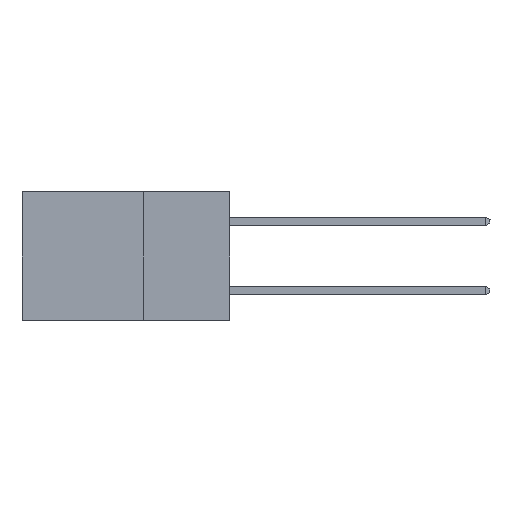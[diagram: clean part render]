
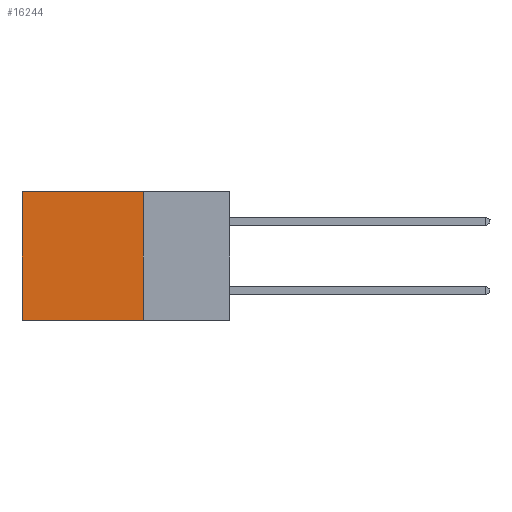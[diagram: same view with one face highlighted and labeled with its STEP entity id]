
A CAD part, left-side view. The second image highlights one B-rep face of the part: STEP entity #16244.
In plain terms, the highlighted planar face has unit normal (-1, 0, 0).
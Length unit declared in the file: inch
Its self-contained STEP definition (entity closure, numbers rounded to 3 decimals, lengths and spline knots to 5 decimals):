
#176 = FACE_OUTER_BOUND ( 'NONE', #15796, .T. ) ;
#634 = VECTOR ( 'NONE', #16103, 39.37008 ) ;
#1981 = ORIENTED_EDGE ( 'NONE', *, *, #16188, .T. ) ;
#2807 = CARTESIAN_POINT ( 'NONE',  ( 0.2615, 0.25, 0. ) ) ;
#4240 = DIRECTION ( 'NONE',  ( 1., 0., 0. ) ) ;
#4374 = LINE ( 'NONE', #25330, #18898 ) ;
#4398 = EDGE_CURVE ( 'NONE', #14959, #13245, #10798, .T. ) ;
#4508 = PLANE ( 'NONE',  #19746 ) ;
#4980 = DIRECTION ( 'NONE',  ( 0., 0., -1. ) ) ;
#7429 = VECTOR ( 'NONE', #11198, 39.37008 ) ;
#8577 = CARTESIAN_POINT ( 'NONE',  ( 0.2615, 0.6, 0. ) ) ;
#9911 = CARTESIAN_POINT ( 'NONE',  ( 0.2615, 0.25, -0.37 ) ) ;
#9934 = ORIENTED_EDGE ( 'NONE', *, *, #12156, .F. ) ;
#10798 = LINE ( 'NONE', #2807, #7429 ) ;
#11198 = DIRECTION ( 'NONE',  ( 0., 1., 0. ) ) ;
#12156 = EDGE_CURVE ( 'NONE', #14094, #20767, #14093, .T. ) ;
#12673 = ORIENTED_EDGE ( 'NONE', *, *, #17372, .F. ) ;
#13245 = VERTEX_POINT ( 'NONE', #8577 ) ;
#14093 = LINE ( 'NONE', #9911, #634 ) ;
#14094 = VERTEX_POINT ( 'NONE', #14123 ) ;
#14123 = CARTESIAN_POINT ( 'NONE',  ( 0.2615, 0.25, -0.37 ) ) ;
#14959 = VERTEX_POINT ( 'NONE', #16953 ) ;
#15796 = EDGE_LOOP ( 'NONE', ( #1981, #9934, #12673, #23263 ) ) ;
#16103 = DIRECTION ( 'NONE',  ( 0., 1., 0. ) ) ;
#16188 = EDGE_CURVE ( 'NONE', #13245, #20767, #4374, .T. ) ;
#16244 = ADVANCED_FACE ( 'NONE', ( #176 ), #4508, .F. ) ;
#16953 = CARTESIAN_POINT ( 'NONE',  ( 0.2615, 0.25, 0. ) ) ;
#17350 = CARTESIAN_POINT ( 'NONE',  ( 0.2615, 0.6, -0.37 ) ) ;
#17372 = EDGE_CURVE ( 'NONE', #14959, #14094, #25953, .T. ) ;
#18898 = VECTOR ( 'NONE', #23164, 39.37008 ) ;
#19746 = AXIS2_PLACEMENT_3D ( 'NONE', #25198, #4240, #21257 ) ;
#20767 = VERTEX_POINT ( 'NONE', #17350 ) ;
#21257 = DIRECTION ( 'NONE',  ( 0., 0., -1. ) ) ;
#21515 = VECTOR ( 'NONE', #4980, 39.37008 ) ;
#23164 = DIRECTION ( 'NONE',  ( 0., 0., -1. ) ) ;
#23263 = ORIENTED_EDGE ( 'NONE', *, *, #4398, .T. ) ;
#25198 = CARTESIAN_POINT ( 'NONE',  ( 0.2615, 0.25, -0.37 ) ) ;
#25330 = CARTESIAN_POINT ( 'NONE',  ( 0.2615, 0.6, -0.37 ) ) ;
#25406 = CARTESIAN_POINT ( 'NONE',  ( 0.2615, 0.25, -0.37 ) ) ;
#25953 = LINE ( 'NONE', #25406, #21515 ) ;
